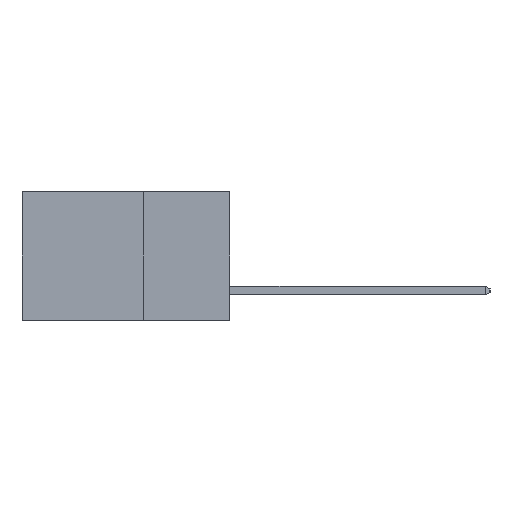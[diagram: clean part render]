
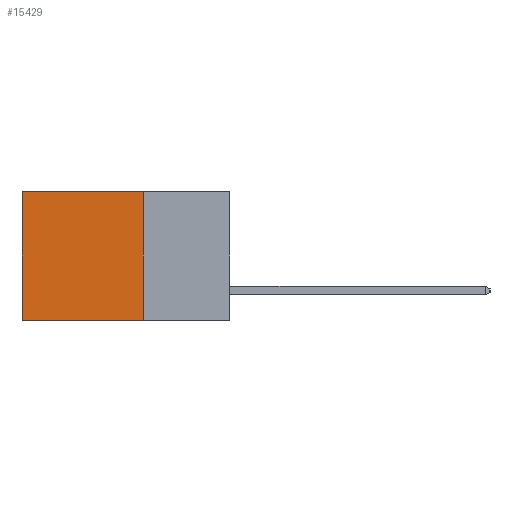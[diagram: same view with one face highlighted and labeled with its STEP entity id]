
A CAD part, left-side view. The second image highlights one B-rep face of the part: STEP entity #15429.
In plain terms, the highlighted planar face has unit normal (-1, 0, 0).
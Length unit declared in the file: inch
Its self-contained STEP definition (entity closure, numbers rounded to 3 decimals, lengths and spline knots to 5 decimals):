
#442 = CARTESIAN_POINT ( 'NONE',  ( 0.298, 0.6, -0.37 ) ) ;
#657 = CARTESIAN_POINT ( 'NONE',  ( 0.298, 0.25, 0. ) ) ;
#1388 = VERTEX_POINT ( 'NONE', #16821 ) ;
#2137 = EDGE_CURVE ( 'NONE', #12980, #1388, #5366, .T. ) ;
#4209 = EDGE_LOOP ( 'NONE', ( #22860, #12937, #10187, #19940 ) ) ;
#4420 = VECTOR ( 'NONE', #15426, 39.37008 ) ;
#4508 = EDGE_CURVE ( 'NONE', #8866, #13354, #13720, .T. ) ;
#4790 = VECTOR ( 'NONE', #7266, 39.37008 ) ;
#5366 = LINE ( 'NONE', #23113, #4790 ) ;
#6115 = AXIS2_PLACEMENT_3D ( 'NONE', #8482, #21155, #10303 ) ;
#7266 = DIRECTION ( 'NONE',  ( 0., 0., -1. ) ) ;
#7455 = EDGE_CURVE ( 'NONE', #1388, #13354, #23446, .T. ) ;
#8482 = CARTESIAN_POINT ( 'NONE',  ( 0.298, 0.25, 0. ) ) ;
#8866 = VERTEX_POINT ( 'NONE', #11532 ) ;
#10187 = ORIENTED_EDGE ( 'NONE', *, *, #2137, .F. ) ;
#10303 = DIRECTION ( 'NONE',  ( 0., 0., -1. ) ) ;
#11532 = CARTESIAN_POINT ( 'NONE',  ( 0.298, 0.6, 0. ) ) ;
#11743 = FACE_OUTER_BOUND ( 'NONE', #4209, .T. ) ;
#12150 = DIRECTION ( 'NONE',  ( 0., 0., -1. ) ) ;
#12937 = ORIENTED_EDGE ( 'NONE', *, *, #7455, .F. ) ;
#12980 = VERTEX_POINT ( 'NONE', #17680 ) ;
#13094 = DIRECTION ( 'NONE',  ( 0., 1., 0. ) ) ;
#13314 = VECTOR ( 'NONE', #13094, 39.37008 ) ;
#13354 = VERTEX_POINT ( 'NONE', #442 ) ;
#13720 = LINE ( 'NONE', #14125, #22722 ) ;
#14125 = CARTESIAN_POINT ( 'NONE',  ( 0.298, 0.6, 0. ) ) ;
#15426 = DIRECTION ( 'NONE',  ( 0., 1., 0. ) ) ;
#15429 = ADVANCED_FACE ( 'NONE', ( #11743 ), #15774, .F. ) ;
#15774 = PLANE ( 'NONE',  #6115 ) ;
#16359 = EDGE_CURVE ( 'NONE', #12980, #8866, #17721, .T. ) ;
#16774 = CARTESIAN_POINT ( 'NONE',  ( 0.298, 0.25, -0.37 ) ) ;
#16821 = CARTESIAN_POINT ( 'NONE',  ( 0.298, 0.25, -0.37 ) ) ;
#17680 = CARTESIAN_POINT ( 'NONE',  ( 0.298, 0.25, 0. ) ) ;
#17721 = LINE ( 'NONE', #657, #4420 ) ;
#19940 = ORIENTED_EDGE ( 'NONE', *, *, #16359, .T. ) ;
#21155 = DIRECTION ( 'NONE',  ( 1., 0., 0. ) ) ;
#22722 = VECTOR ( 'NONE', #12150, 39.37008 ) ;
#22860 = ORIENTED_EDGE ( 'NONE', *, *, #4508, .T. ) ;
#23113 = CARTESIAN_POINT ( 'NONE',  ( 0.298, 0.25, 0. ) ) ;
#23446 = LINE ( 'NONE', #16774, #13314 ) ;
